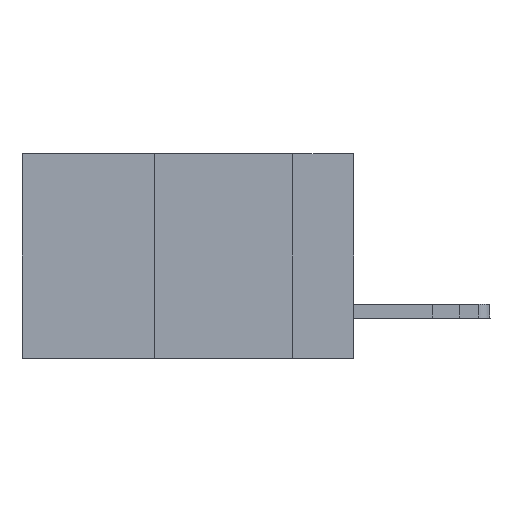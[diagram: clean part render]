
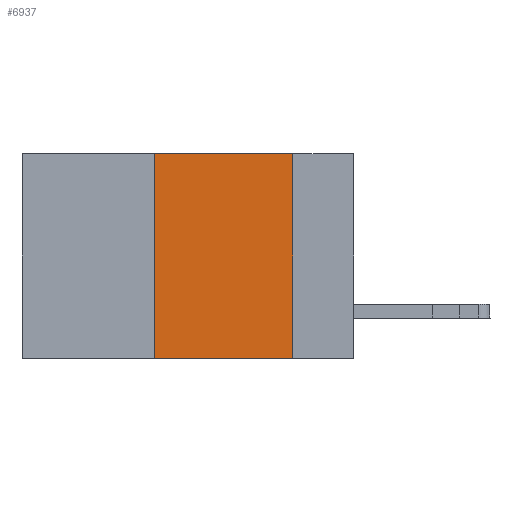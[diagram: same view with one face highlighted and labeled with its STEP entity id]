
A CAD part, left-side view. The second image highlights one B-rep face of the part: STEP entity #6937.
In plain terms, the highlighted planar face has unit normal (-1, 0, 0).
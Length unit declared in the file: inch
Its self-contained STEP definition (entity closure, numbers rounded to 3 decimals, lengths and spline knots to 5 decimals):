
#261 = EDGE_CURVE ( 'NONE', #16083, #3552, #6381, .T. ) ;
#591 = EDGE_CURVE ( 'NONE', #23010, #3552, #9291, .T. ) ;
#1706 = DIRECTION ( 'NONE',  ( 0., 0., -1. ) ) ;
#3045 = EDGE_LOOP ( 'NONE', ( #9334, #22058, #6083, #15412 ) ) ;
#3552 = VERTEX_POINT ( 'NONE', #21332 ) ;
#3699 = CARTESIAN_POINT ( 'NONE',  ( 0., 0.6, 0. ) ) ;
#5774 = LINE ( 'NONE', #3699, #20049 ) ;
#6074 = CARTESIAN_POINT ( 'NONE',  ( 0., 0.36, 0. ) ) ;
#6083 = ORIENTED_EDGE ( 'NONE', *, *, #10389, .F. ) ;
#6381 = LINE ( 'NONE', #15041, #6959 ) ;
#6937 = ADVANCED_FACE ( 'NONE', ( #8256 ), #11078, .F. ) ;
#6959 = VECTOR ( 'NONE', #21552, 39.37008 ) ;
#7781 = DIRECTION ( 'NONE',  ( 0., 0., 1. ) ) ;
#8008 = AXIS2_PLACEMENT_3D ( 'NONE', #18459, #12954, #1706 ) ;
#8256 = FACE_OUTER_BOUND ( 'NONE', #3045, .T. ) ;
#9108 = VECTOR ( 'NONE', #7781, 39.37008 ) ;
#9291 = LINE ( 'NONE', #17948, #19200 ) ;
#9334 = ORIENTED_EDGE ( 'NONE', *, *, #591, .F. ) ;
#10389 = EDGE_CURVE ( 'NONE', #16083, #19051, #14067, .T. ) ;
#11078 = PLANE ( 'NONE',  #8008 ) ;
#11922 = CARTESIAN_POINT ( 'NONE',  ( 0., 0.11, 0. ) ) ;
#12501 = EDGE_CURVE ( 'NONE', #19051, #23010, #5774, .T. ) ;
#12954 = DIRECTION ( 'NONE',  ( 1., 0., 0. ) ) ;
#14067 = LINE ( 'NONE', #22562, #9108 ) ;
#15041 = CARTESIAN_POINT ( 'NONE',  ( 0., 0.6, -0.37 ) ) ;
#15412 = ORIENTED_EDGE ( 'NONE', *, *, #261, .T. ) ;
#16083 = VERTEX_POINT ( 'NONE', #21095 ) ;
#17923 = DIRECTION ( 'NONE',  ( 0., 0., -1. ) ) ;
#17948 = CARTESIAN_POINT ( 'NONE',  ( 0., 0.11, 0. ) ) ;
#18459 = CARTESIAN_POINT ( 'NONE',  ( 0., 0.6, 0. ) ) ;
#19051 = VERTEX_POINT ( 'NONE', #6074 ) ;
#19200 = VECTOR ( 'NONE', #17923, 39.37008 ) ;
#20049 = VECTOR ( 'NONE', #20385, 39.37008 ) ;
#20385 = DIRECTION ( 'NONE',  ( 0., -1., 0. ) ) ;
#21095 = CARTESIAN_POINT ( 'NONE',  ( 0., 0.36, -0.37 ) ) ;
#21332 = CARTESIAN_POINT ( 'NONE',  ( 0., 0.11, -0.37 ) ) ;
#21552 = DIRECTION ( 'NONE',  ( 0., -1., 0. ) ) ;
#22058 = ORIENTED_EDGE ( 'NONE', *, *, #12501, .F. ) ;
#22562 = CARTESIAN_POINT ( 'NONE',  ( 0., 0.36, 0. ) ) ;
#23010 = VERTEX_POINT ( 'NONE', #11922 ) ;
